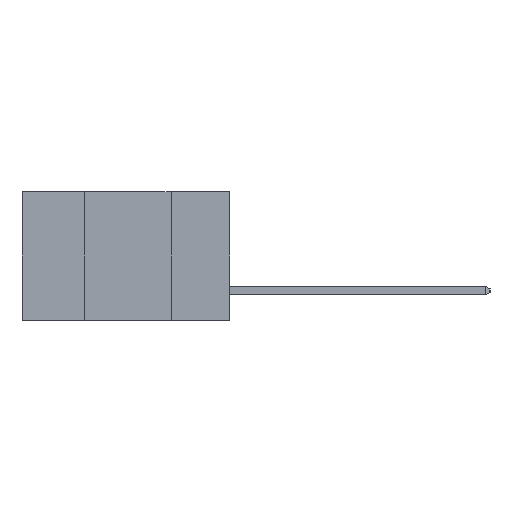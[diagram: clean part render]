
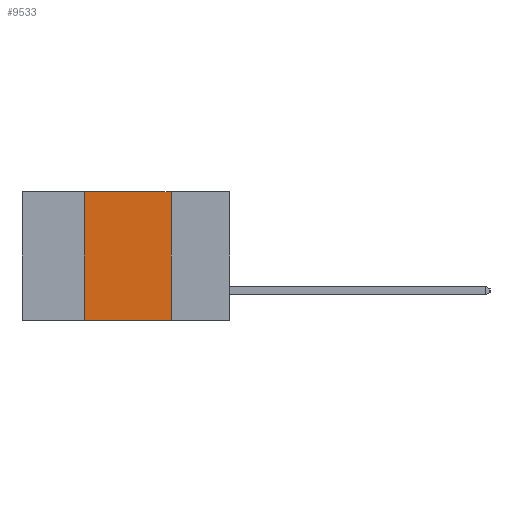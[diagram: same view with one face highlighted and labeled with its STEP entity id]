
A CAD part, left-side view. The second image highlights one B-rep face of the part: STEP entity #9533.
In plain terms, the highlighted planar face has unit normal (-1, 0, 0).
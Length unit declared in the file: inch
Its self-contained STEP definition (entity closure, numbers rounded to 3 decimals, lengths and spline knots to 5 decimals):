
#865 = EDGE_LOOP ( 'NONE', ( #17760, #19361, #21513, #11923 ) ) ;
#1629 = VERTEX_POINT ( 'NONE', #14913 ) ;
#1933 = CARTESIAN_POINT ( 'NONE',  ( 0., 0.17, 0. ) ) ;
#2583 = CARTESIAN_POINT ( 'NONE',  ( 0., 0.17, 0. ) ) ;
#3144 = DIRECTION ( 'NONE',  ( 0., 0., 1. ) ) ;
#4267 = DIRECTION ( 'NONE',  ( 0., 0., -1. ) ) ;
#4317 = CARTESIAN_POINT ( 'NONE',  ( 0., 0.17, -0.37 ) ) ;
#4523 = DIRECTION ( 'NONE',  ( 0., 0., -1. ) ) ;
#4535 = EDGE_CURVE ( 'NONE', #13413, #4875, #21249, .T. ) ;
#4875 = VERTEX_POINT ( 'NONE', #4317 ) ;
#5215 = LINE ( 'NONE', #19495, #9172 ) ;
#5491 = DIRECTION ( 'NONE',  ( 0., -1., 0. ) ) ;
#6334 = CARTESIAN_POINT ( 'NONE',  ( 0., 0.42, -0.37 ) ) ;
#7566 = LINE ( 'NONE', #2583, #21278 ) ;
#9030 = EDGE_CURVE ( 'NONE', #13413, #1629, #12203, .T. ) ;
#9122 = VECTOR ( 'NONE', #5491, 39.37008 ) ;
#9172 = VECTOR ( 'NONE', #11233, 39.37008 ) ;
#9483 = CARTESIAN_POINT ( 'NONE',  ( 0., 0.6, 0. ) ) ;
#9533 = ADVANCED_FACE ( 'NONE', ( #9662 ), #12739, .F. ) ;
#9579 = EDGE_CURVE ( 'NONE', #1629, #13539, #5215, .T. ) ;
#9662 = FACE_OUTER_BOUND ( 'NONE', #865, .T. ) ;
#10096 = EDGE_CURVE ( 'NONE', #13539, #4875, #7566, .T. ) ;
#11233 = DIRECTION ( 'NONE',  ( 0., -1., 0. ) ) ;
#11923 = ORIENTED_EDGE ( 'NONE', *, *, #4535, .T. ) ;
#12203 = LINE ( 'NONE', #16396, #20564 ) ;
#12218 = CARTESIAN_POINT ( 'NONE',  ( 0., 0.6, -0.37 ) ) ;
#12739 = PLANE ( 'NONE',  #21404 ) ;
#13413 = VERTEX_POINT ( 'NONE', #6334 ) ;
#13539 = VERTEX_POINT ( 'NONE', #1933 ) ;
#14433 = DIRECTION ( 'NONE',  ( 1., 0., 0. ) ) ;
#14913 = CARTESIAN_POINT ( 'NONE',  ( 0., 0.42, 0. ) ) ;
#16396 = CARTESIAN_POINT ( 'NONE',  ( 0., 0.42, 0. ) ) ;
#17760 = ORIENTED_EDGE ( 'NONE', *, *, #10096, .F. ) ;
#19361 = ORIENTED_EDGE ( 'NONE', *, *, #9579, .F. ) ;
#19495 = CARTESIAN_POINT ( 'NONE',  ( 0., 0.6, 0. ) ) ;
#20564 = VECTOR ( 'NONE', #3144, 39.37008 ) ;
#21249 = LINE ( 'NONE', #12218, #9122 ) ;
#21278 = VECTOR ( 'NONE', #4267, 39.37008 ) ;
#21404 = AXIS2_PLACEMENT_3D ( 'NONE', #9483, #14433, #4523 ) ;
#21513 = ORIENTED_EDGE ( 'NONE', *, *, #9030, .F. ) ;
